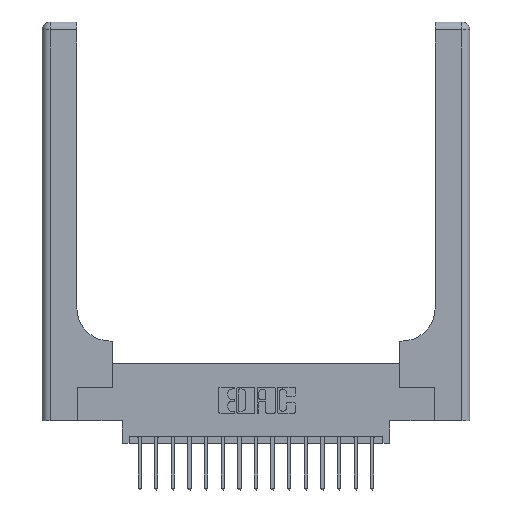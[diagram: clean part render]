
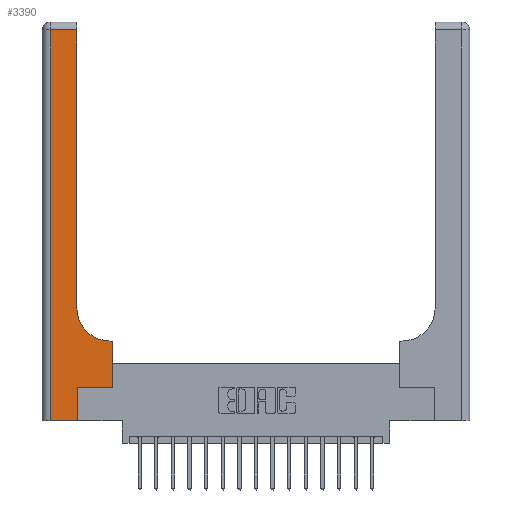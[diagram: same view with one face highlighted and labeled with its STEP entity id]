
A CAD part, top view. The second image highlights one B-rep face of the part: STEP entity #3390.
In plain terms, the highlighted planar face has unit normal (0, 0, 1).
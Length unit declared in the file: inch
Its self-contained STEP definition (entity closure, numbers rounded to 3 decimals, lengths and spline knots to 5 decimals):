
#187 = EDGE_CURVE ( 'NONE', #3163, #10548, #7371, .T. ) ;
#453 = CARTESIAN_POINT ( 'NONE',  ( 0.528, 0.25, 0.37 ) ) ;
#822 = ORIENTED_EDGE ( 'NONE', *, *, #187, .T. ) ;
#1329 = EDGE_CURVE ( 'NONE', #12006, #2054, #1957, .T. ) ;
#1338 = CARTESIAN_POINT ( 'NONE',  ( 0.265, 0.25, 0.37 ) ) ;
#1450 = VECTOR ( 'NONE', #12508, 39.37008 ) ;
#1635 = CARTESIAN_POINT ( 'NONE',  ( 0.26, 0.85, 0.37 ) ) ;
#1780 = CARTESIAN_POINT ( 'NONE',  ( 0.528, 0.25, 0.37 ) ) ;
#1838 = EDGE_CURVE ( 'NONE', #10548, #7655, #14943, .T. ) ;
#1957 = LINE ( 'NONE', #4979, #2713 ) ;
#2054 = VERTEX_POINT ( 'NONE', #11530 ) ;
#2713 = VECTOR ( 'NONE', #17907, 39.37008 ) ;
#3163 = VERTEX_POINT ( 'NONE', #18367 ) ;
#3205 = CARTESIAN_POINT ( 'NONE',  ( 0.26, 3., 0.37 ) ) ;
#3212 = LINE ( 'NONE', #9411, #8682 ) ;
#3238 = DIRECTION ( 'NONE',  ( 1., 0., 0. ) ) ;
#3390 = ADVANCED_FACE ( 'NONE', ( #7832 ), #12315, .F. ) ;
#3548 = ORIENTED_EDGE ( 'NONE', *, *, #9754, .T. ) ;
#3859 = LINE ( 'NONE', #14462, #15585 ) ;
#4129 = EDGE_CURVE ( 'NONE', #7655, #12006, #18888, .T. ) ;
#4265 = AXIS2_PLACEMENT_3D ( 'NONE', #14802, #7413, #3238 ) ;
#4645 = DIRECTION ( 'NONE',  ( -1., 0., 0. ) ) ;
#4979 = CARTESIAN_POINT ( 'NONE',  ( 0.06, 3., 0.37 ) ) ;
#4999 = ORIENTED_EDGE ( 'NONE', *, *, #11941, .T. ) ;
#5367 = VECTOR ( 'NONE', #8404, 39.37008 ) ;
#5515 = EDGE_CURVE ( 'NONE', #2054, #6564, #15531, .T. ) ;
#6460 = CARTESIAN_POINT ( 'NONE',  ( 0.26, 2.94, 0.37 ) ) ;
#6564 = VERTEX_POINT ( 'NONE', #7862 ) ;
#6577 = EDGE_CURVE ( 'NONE', #6564, #17017, #3212, .T. ) ;
#6845 = VECTOR ( 'NONE', #7023, 39.37008 ) ;
#7023 = DIRECTION ( 'NONE',  ( -1., 0., 0. ) ) ;
#7062 = CARTESIAN_POINT ( 'NONE',  ( 0.06, 2.94, 0.37 ) ) ;
#7371 = CIRCLE ( 'NONE', #4265, 0.25 ) ;
#7413 = DIRECTION ( 'NONE',  ( 0., 0., -1. ) ) ;
#7426 = CARTESIAN_POINT ( 'NONE',  ( 0.528, 0.6, 0.37 ) ) ;
#7454 = CARTESIAN_POINT ( 'NONE',  ( 0., 3., 0.37 ) ) ;
#7655 = VERTEX_POINT ( 'NONE', #6460 ) ;
#7832 = FACE_OUTER_BOUND ( 'NONE', #11115, .T. ) ;
#7862 = CARTESIAN_POINT ( 'NONE',  ( 0.265, 0., 0.37 ) ) ;
#8250 = VERTEX_POINT ( 'NONE', #7426 ) ;
#8327 = DIRECTION ( 'NONE',  ( 1., 0., 0. ) ) ;
#8404 = DIRECTION ( 'NONE',  ( 1., 0., 0. ) ) ;
#8469 = CARTESIAN_POINT ( 'NONE',  ( 0., 2.94, 0.37 ) ) ;
#8682 = VECTOR ( 'NONE', #11956, 39.37008 ) ;
#8860 = DIRECTION ( 'NONE',  ( 0., 1., 0. ) ) ;
#9309 = EDGE_CURVE ( 'NONE', #8250, #3163, #3859, .T. ) ;
#9411 = CARTESIAN_POINT ( 'NONE',  ( 0.265, 0., 0.37 ) ) ;
#9623 = ORIENTED_EDGE ( 'NONE', *, *, #6577, .T. ) ;
#9754 = EDGE_CURVE ( 'NONE', #14278, #8250, #10509, .T. ) ;
#10509 = LINE ( 'NONE', #1780, #12199 ) ;
#10548 = VERTEX_POINT ( 'NONE', #1635 ) ;
#10832 = ORIENTED_EDGE ( 'NONE', *, *, #4129, .T. ) ;
#11115 = EDGE_LOOP ( 'NONE', ( #19192, #10832, #15066, #18105, #9623, #4999, #3548, #13778, #822 ) ) ;
#11134 = VECTOR ( 'NONE', #8327, 39.37008 ) ;
#11530 = CARTESIAN_POINT ( 'NONE',  ( 0.06, 0., 0.37 ) ) ;
#11941 = EDGE_CURVE ( 'NONE', #17017, #14278, #14446, .T. ) ;
#11956 = DIRECTION ( 'NONE',  ( 0., 1., 0. ) ) ;
#12006 = VERTEX_POINT ( 'NONE', #7062 ) ;
#12199 = VECTOR ( 'NONE', #8860, 39.37008 ) ;
#12315 = PLANE ( 'NONE',  #16677 ) ;
#12508 = DIRECTION ( 'NONE',  ( 0., 1., 0. ) ) ;
#13778 = ORIENTED_EDGE ( 'NONE', *, *, #9309, .T. ) ;
#14278 = VERTEX_POINT ( 'NONE', #453 ) ;
#14446 = LINE ( 'NONE', #15700, #5367 ) ;
#14462 = CARTESIAN_POINT ( 'NONE',  ( 0.26, 0.6, 0.37 ) ) ;
#14802 = CARTESIAN_POINT ( 'NONE',  ( 0.51, 0.85, 0.37 ) ) ;
#14943 = LINE ( 'NONE', #3205, #1450 ) ;
#15066 = ORIENTED_EDGE ( 'NONE', *, *, #1329, .T. ) ;
#15117 = DIRECTION ( 'NONE',  ( 0., 0., -1. ) ) ;
#15329 = CARTESIAN_POINT ( 'NONE',  ( 0., 0., 0.37 ) ) ;
#15531 = LINE ( 'NONE', #15329, #11134 ) ;
#15585 = VECTOR ( 'NONE', #18837, 39.37008 ) ;
#15700 = CARTESIAN_POINT ( 'NONE',  ( 0.265, 0.25, 0.37 ) ) ;
#16677 = AXIS2_PLACEMENT_3D ( 'NONE', #7454, #15117, #4645 ) ;
#17017 = VERTEX_POINT ( 'NONE', #1338 ) ;
#17907 = DIRECTION ( 'NONE',  ( 0., -1., 0. ) ) ;
#18105 = ORIENTED_EDGE ( 'NONE', *, *, #5515, .T. ) ;
#18367 = CARTESIAN_POINT ( 'NONE',  ( 0.51, 0.6, 0.37 ) ) ;
#18837 = DIRECTION ( 'NONE',  ( -1., 0., 0. ) ) ;
#18888 = LINE ( 'NONE', #8469, #6845 ) ;
#19192 = ORIENTED_EDGE ( 'NONE', *, *, #1838, .T. ) ;
